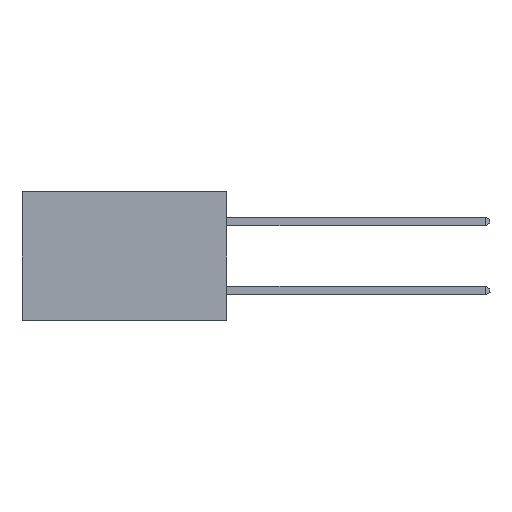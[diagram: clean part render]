
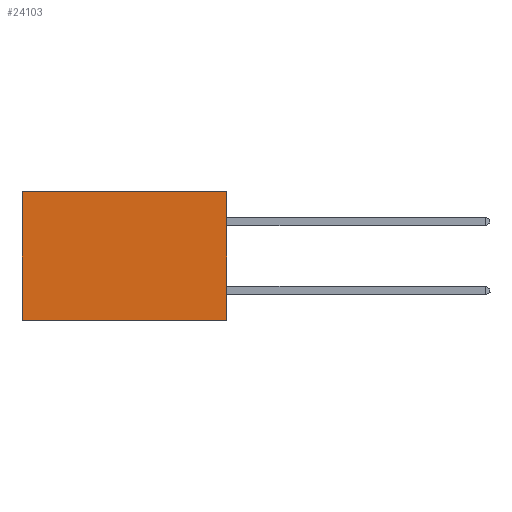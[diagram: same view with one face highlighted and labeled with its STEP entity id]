
A CAD part, left-side view. The second image highlights one B-rep face of the part: STEP entity #24103.
In plain terms, the highlighted planar face has unit normal (-1, 0, 0).
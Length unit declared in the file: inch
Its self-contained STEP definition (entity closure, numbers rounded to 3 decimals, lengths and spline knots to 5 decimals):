
#252 = VERTEX_POINT ( 'NONE', #15363 ) ;
#449 = CARTESIAN_POINT ( 'NONE',  ( 0.277, 0., -0.37 ) ) ;
#3202 = DIRECTION ( 'NONE',  ( 0., 1., 0. ) ) ;
#4597 = CARTESIAN_POINT ( 'NONE',  ( 0.277, 0., -0.37 ) ) ;
#5159 = CARTESIAN_POINT ( 'NONE',  ( 0.277, 0., 0. ) ) ;
#6062 = CARTESIAN_POINT ( 'NONE',  ( 0.277, 0.59, -0.37 ) ) ;
#6615 = DIRECTION ( 'NONE',  ( 1., 0., 0. ) ) ;
#6697 = DIRECTION ( 'NONE',  ( 0., 1., 0. ) ) ;
#6920 = CARTESIAN_POINT ( 'NONE',  ( 0.277, 0., -0.37 ) ) ;
#7185 = VECTOR ( 'NONE', #3202, 39.37008 ) ;
#7287 = VECTOR ( 'NONE', #25208, 39.37008 ) ;
#7921 = LINE ( 'NONE', #23236, #7287 ) ;
#8230 = AXIS2_PLACEMENT_3D ( 'NONE', #4597, #6615, #20573 ) ;
#9296 = LINE ( 'NONE', #6062, #14598 ) ;
#10212 = EDGE_CURVE ( 'NONE', #12562, #24429, #15188, .T. ) ;
#11464 = CARTESIAN_POINT ( 'NONE',  ( 0.277, 0.59, -0.37 ) ) ;
#12562 = VERTEX_POINT ( 'NONE', #6920 ) ;
#13076 = LINE ( 'NONE', #5159, #7185 ) ;
#14528 = PLANE ( 'NONE',  #8230 ) ;
#14598 = VECTOR ( 'NONE', #25836, 39.37008 ) ;
#15188 = LINE ( 'NONE', #449, #21150 ) ;
#15204 = EDGE_CURVE ( 'NONE', #252, #20918, #13076, .T. ) ;
#15363 = CARTESIAN_POINT ( 'NONE',  ( 0.277, 0., 0. ) ) ;
#17625 = CARTESIAN_POINT ( 'NONE',  ( 0.277, 0.59, 0. ) ) ;
#19311 = ORIENTED_EDGE ( 'NONE', *, *, #15204, .T. ) ;
#19616 = ORIENTED_EDGE ( 'NONE', *, *, #10212, .F. ) ;
#19741 = EDGE_LOOP ( 'NONE', ( #24333, #19616, #21264, #19311 ) ) ;
#20573 = DIRECTION ( 'NONE',  ( 0., 0., -1. ) ) ;
#20918 = VERTEX_POINT ( 'NONE', #17625 ) ;
#21150 = VECTOR ( 'NONE', #6697, 39.37008 ) ;
#21264 = ORIENTED_EDGE ( 'NONE', *, *, #22779, .F. ) ;
#22407 = FACE_OUTER_BOUND ( 'NONE', #19741, .T. ) ;
#22779 = EDGE_CURVE ( 'NONE', #252, #12562, #7921, .T. ) ;
#23236 = CARTESIAN_POINT ( 'NONE',  ( 0.277, 0., -0.37 ) ) ;
#24103 = ADVANCED_FACE ( 'NONE', ( #22407 ), #14528, .F. ) ;
#24333 = ORIENTED_EDGE ( 'NONE', *, *, #24628, .T. ) ;
#24429 = VERTEX_POINT ( 'NONE', #11464 ) ;
#24628 = EDGE_CURVE ( 'NONE', #20918, #24429, #9296, .T. ) ;
#25208 = DIRECTION ( 'NONE',  ( 0., 0., -1. ) ) ;
#25836 = DIRECTION ( 'NONE',  ( 0., 0., -1. ) ) ;
